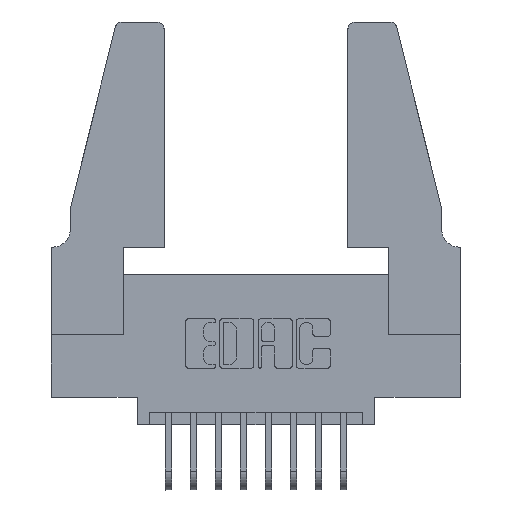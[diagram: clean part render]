
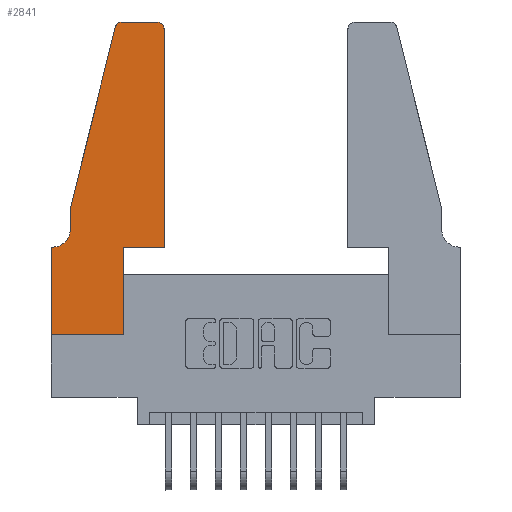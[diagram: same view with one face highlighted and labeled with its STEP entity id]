
A CAD part, top view. The second image highlights one B-rep face of the part: STEP entity #2841.
In plain terms, the highlighted planar face has unit normal (0, 0, 1).
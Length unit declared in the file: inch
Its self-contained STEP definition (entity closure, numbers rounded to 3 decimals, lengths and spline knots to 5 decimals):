
#723 = VECTOR ( 'NONE', #9233, 39.37008 ) ;
#828 = VECTOR ( 'NONE', #11654, 39.37008 ) ;
#869 = CIRCLE ( 'NONE', #11562, 0.03 ) ;
#1034 = ORIENTED_EDGE ( 'NONE', *, *, #3690, .T. ) ;
#1096 = LINE ( 'NONE', #11215, #3461 ) ;
#1351 = LINE ( 'NONE', #8799, #9083 ) ;
#1380 = VERTEX_POINT ( 'NONE', #10711 ) ;
#1690 = CARTESIAN_POINT ( 'NONE',  ( 0.284, 1.25, 0.37 ) ) ;
#1746 = DIRECTION ( 'NONE',  ( -0.239, -0.971, 0. ) ) ;
#1949 = EDGE_CURVE ( 'NONE', #9442, #6751, #12990, .T. ) ;
#1983 = ORIENTED_EDGE ( 'NONE', *, *, #2081, .T. ) ;
#2054 = DIRECTION ( 'NONE',  ( 0., -1., 0. ) ) ;
#2081 = EDGE_CURVE ( 'NONE', #1380, #12666, #1096, .T. ) ;
#2166 = CIRCLE ( 'NONE', #6878, 0.07 ) ;
#2306 = EDGE_CURVE ( 'NONE', #6751, #10962, #8986, .T. ) ;
#2485 = ORIENTED_EDGE ( 'NONE', *, *, #8455, .T. ) ;
#2583 = CARTESIAN_POINT ( 'NONE',  ( 0.0755, 0.5, 0.37 ) ) ;
#2841 = ADVANCED_FACE ( 'NONE', ( #11293 ), #7544, .T. ) ;
#2969 = CARTESIAN_POINT ( 'NONE',  ( 0.25487, 1.22718, 0.37 ) ) ;
#3045 = DIRECTION ( 'NONE',  ( 0., 0., 1. ) ) ;
#3070 = DIRECTION ( 'NONE',  ( 1., 0., 0. ) ) ;
#3196 = CARTESIAN_POINT ( 'NONE',  ( 0., 0., 0.37 ) ) ;
#3461 = VECTOR ( 'NONE', #5456, 39.37008 ) ;
#3517 = LINE ( 'NONE', #5645, #828 ) ;
#3563 = LINE ( 'NONE', #11469, #6270 ) ;
#3657 = ORIENTED_EDGE ( 'NONE', *, *, #12980, .T. ) ;
#3690 = EDGE_CURVE ( 'NONE', #10962, #5309, #10630, .T. ) ;
#3925 = ORIENTED_EDGE ( 'NONE', *, *, #8262, .T. ) ;
#4111 = LINE ( 'NONE', #9094, #5888 ) ;
#4258 = EDGE_CURVE ( 'NONE', #6337, #6725, #1351, .T. ) ;
#4271 = CARTESIAN_POINT ( 'NONE',  ( 0.2865, 0.35, 0.37 ) ) ;
#4336 = CARTESIAN_POINT ( 'NONE',  ( 0.4205, 1.25, 0.37 ) ) ;
#4360 = ORIENTED_EDGE ( 'NONE', *, *, #10909, .T. ) ;
#4433 = CARTESIAN_POINT ( 'NONE',  ( 0.0055, 0.42, 0.37 ) ) ;
#4594 = AXIS2_PLACEMENT_3D ( 'NONE', #4889, #11883, #5928 ) ;
#4619 = CARTESIAN_POINT ( 'NONE',  ( 0.284, 1.22, 0.37 ) ) ;
#4742 = LINE ( 'NONE', #12238, #9742 ) ;
#4752 = EDGE_CURVE ( 'NONE', #5309, #11481, #3563, .T. ) ;
#4889 = CARTESIAN_POINT ( 'NONE',  ( 0.4205, 1.22, 0.37 ) ) ;
#5309 = VERTEX_POINT ( 'NONE', #4336 ) ;
#5336 = CARTESIAN_POINT ( 'NONE',  ( 0.4505, 0.35, 0.37 ) ) ;
#5456 = DIRECTION ( 'NONE',  ( -1., 0., 0. ) ) ;
#5479 = DIRECTION ( 'NONE',  ( -1., 0., 0. ) ) ;
#5645 = CARTESIAN_POINT ( 'NONE',  ( 0.2865, 0.35, 0.37 ) ) ;
#5654 = DIRECTION ( 'NONE',  ( 1., 0., 0. ) ) ;
#5888 = VECTOR ( 'NONE', #2054, 39.37008 ) ;
#5928 = DIRECTION ( 'NONE',  ( 1., 0., 0. ) ) ;
#6088 = ORIENTED_EDGE ( 'NONE', *, *, #12297, .T. ) ;
#6270 = VECTOR ( 'NONE', #9468, 39.37008 ) ;
#6309 = VECTOR ( 'NONE', #7328, 39.37008 ) ;
#6337 = VERTEX_POINT ( 'NONE', #2969 ) ;
#6725 = VERTEX_POINT ( 'NONE', #2583 ) ;
#6751 = VERTEX_POINT ( 'NONE', #11615 ) ;
#6762 = CARTESIAN_POINT ( 'NONE',  ( 0.2865, 0., 0.37 ) ) ;
#6878 = AXIS2_PLACEMENT_3D ( 'NONE', #4433, #11452, #5479 ) ;
#7282 = ORIENTED_EDGE ( 'NONE', *, *, #4752, .T. ) ;
#7328 = DIRECTION ( 'NONE',  ( 0., 1., 0. ) ) ;
#7407 = ORIENTED_EDGE ( 'NONE', *, *, #1949, .T. ) ;
#7539 = CARTESIAN_POINT ( 'NONE',  ( 0., 0.35, 0.37 ) ) ;
#7544 = PLANE ( 'NONE',  #11381 ) ;
#7746 = VECTOR ( 'NONE', #8395, 39.37008 ) ;
#8262 = EDGE_CURVE ( 'NONE', #9451, #9758, #11102, .T. ) ;
#8300 = DIRECTION ( 'NONE',  ( 0., -1., 0. ) ) ;
#8374 = EDGE_CURVE ( 'NONE', #11863, #1380, #2166, .T. ) ;
#8395 = DIRECTION ( 'NONE',  ( 1., 0., 0. ) ) ;
#8455 = EDGE_CURVE ( 'NONE', #11481, #6337, #869, .T. ) ;
#8756 = CARTESIAN_POINT ( 'NONE',  ( 0.4505, 1.22, 0.37 ) ) ;
#8799 = CARTESIAN_POINT ( 'NONE',  ( 0.0755, 0.5, 0.37 ) ) ;
#8986 = LINE ( 'NONE', #5336, #6309 ) ;
#9083 = VECTOR ( 'NONE', #1746, 39.37008 ) ;
#9094 = CARTESIAN_POINT ( 'NONE',  ( 0., 0., 0.37 ) ) ;
#9233 = DIRECTION ( 'NONE',  ( 1., 0., 0. ) ) ;
#9361 = CARTESIAN_POINT ( 'NONE',  ( 0.0755, 0.42, 0.37 ) ) ;
#9442 = VERTEX_POINT ( 'NONE', #4271 ) ;
#9451 = VERTEX_POINT ( 'NONE', #11298 ) ;
#9468 = DIRECTION ( 'NONE',  ( -1., 0., 0. ) ) ;
#9581 = EDGE_LOOP ( 'NONE', ( #7282, #2485, #10246, #3657, #10822, #1983, #6088, #3925, #4360, #7407, #11064, #1034 ) ) ;
#9627 = CARTESIAN_POINT ( 'NONE',  ( 0., 0.35, 0.37 ) ) ;
#9742 = VECTOR ( 'NONE', #8300, 39.37008 ) ;
#9758 = VERTEX_POINT ( 'NONE', #6762 ) ;
#10246 = ORIENTED_EDGE ( 'NONE', *, *, #4258, .T. ) ;
#10319 = CARTESIAN_POINT ( 'NONE',  ( 0.4505, 0.35, 0.37 ) ) ;
#10630 = CIRCLE ( 'NONE', #4594, 0.03 ) ;
#10711 = CARTESIAN_POINT ( 'NONE',  ( 0.0055, 0.35, 0.37 ) ) ;
#10822 = ORIENTED_EDGE ( 'NONE', *, *, #8374, .T. ) ;
#10909 = EDGE_CURVE ( 'NONE', #9758, #9442, #3517, .T. ) ;
#10962 = VERTEX_POINT ( 'NONE', #8756 ) ;
#11064 = ORIENTED_EDGE ( 'NONE', *, *, #2306, .T. ) ;
#11102 = LINE ( 'NONE', #3196, #723 ) ;
#11215 = CARTESIAN_POINT ( 'NONE',  ( 0.0755, 0.35, 0.37 ) ) ;
#11293 = FACE_OUTER_BOUND ( 'NONE', #9581, .T. ) ;
#11298 = CARTESIAN_POINT ( 'NONE',  ( 0., 0., 0.37 ) ) ;
#11381 = AXIS2_PLACEMENT_3D ( 'NONE', #7539, #3045, #3070 ) ;
#11452 = DIRECTION ( 'NONE',  ( 0., 0., -1. ) ) ;
#11469 = CARTESIAN_POINT ( 'NONE',  ( 0.2605, 1.25, 0.37 ) ) ;
#11481 = VERTEX_POINT ( 'NONE', #1690 ) ;
#11562 = AXIS2_PLACEMENT_3D ( 'NONE', #4619, #11616, #5654 ) ;
#11615 = CARTESIAN_POINT ( 'NONE',  ( 0.4505, 0.35, 0.37 ) ) ;
#11616 = DIRECTION ( 'NONE',  ( 0., 0., 1. ) ) ;
#11654 = DIRECTION ( 'NONE',  ( 0., 1., 0. ) ) ;
#11863 = VERTEX_POINT ( 'NONE', #9361 ) ;
#11883 = DIRECTION ( 'NONE',  ( 0., 0., 1. ) ) ;
#12238 = CARTESIAN_POINT ( 'NONE',  ( 0.0755, 0.5, 0.37 ) ) ;
#12297 = EDGE_CURVE ( 'NONE', #12666, #9451, #4111, .T. ) ;
#12666 = VERTEX_POINT ( 'NONE', #9627 ) ;
#12980 = EDGE_CURVE ( 'NONE', #6725, #11863, #4742, .T. ) ;
#12990 = LINE ( 'NONE', #10319, #7746 ) ;
